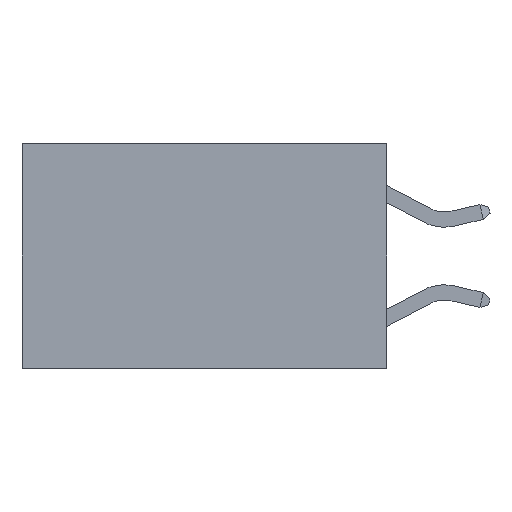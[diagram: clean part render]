
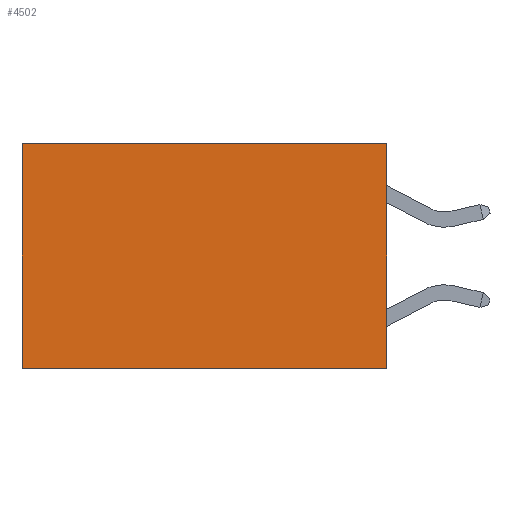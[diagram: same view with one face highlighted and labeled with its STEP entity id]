
A CAD part, left-side view. The second image highlights one B-rep face of the part: STEP entity #4502.
In plain terms, the highlighted planar face has unit normal (-1, 0, 0).
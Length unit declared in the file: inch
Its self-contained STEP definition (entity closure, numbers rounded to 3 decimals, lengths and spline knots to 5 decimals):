
#408 = CARTESIAN_POINT ( 'NONE',  ( 0.2625, 0., 0. ) ) ;
#462 = EDGE_CURVE ( 'NONE', #5724, #863, #1816, .T. ) ;
#844 = CARTESIAN_POINT ( 'NONE',  ( 0.2625, 0., 0. ) ) ;
#863 = VERTEX_POINT ( 'NONE', #2873 ) ;
#1701 = EDGE_CURVE ( 'NONE', #863, #8174, #9578, .T. ) ;
#1816 = LINE ( 'NONE', #408, #9335 ) ;
#1940 = EDGE_LOOP ( 'NONE', ( #2419, #4630, #6530, #8321 ) ) ;
#2263 = DIRECTION ( 'NONE',  ( 0., 0., -1. ) ) ;
#2293 = VECTOR ( 'NONE', #6067, 39.37008 ) ;
#2419 = ORIENTED_EDGE ( 'NONE', *, *, #1701, .T. ) ;
#2873 = CARTESIAN_POINT ( 'NONE',  ( 0.2625, 0.6, 0. ) ) ;
#2953 = VECTOR ( 'NONE', #8441, 39.37008 ) ;
#3237 = LINE ( 'NONE', #4280, #2953 ) ;
#3271 = CARTESIAN_POINT ( 'NONE',  ( 0.2625, 0.6, 0. ) ) ;
#3725 = AXIS2_PLACEMENT_3D ( 'NONE', #9071, #9097, #5076 ) ;
#3895 = CARTESIAN_POINT ( 'NONE',  ( 0.2625, 0., 0. ) ) ;
#3942 = VERTEX_POINT ( 'NONE', #7996 ) ;
#4280 = CARTESIAN_POINT ( 'NONE',  ( 0.2625, 0., -0.37 ) ) ;
#4502 = ADVANCED_FACE ( 'NONE', ( #7821 ), #8464, .F. ) ;
#4533 = LINE ( 'NONE', #3895, #2293 ) ;
#4577 = DIRECTION ( 'NONE',  ( 0., 1., 0. ) ) ;
#4630 = ORIENTED_EDGE ( 'NONE', *, *, #6000, .F. ) ;
#5076 = DIRECTION ( 'NONE',  ( 0., 0., -1. ) ) ;
#5169 = CARTESIAN_POINT ( 'NONE',  ( 0.2625, 0.6, -0.37 ) ) ;
#5724 = VERTEX_POINT ( 'NONE', #844 ) ;
#6000 = EDGE_CURVE ( 'NONE', #3942, #8174, #3237, .T. ) ;
#6064 = VECTOR ( 'NONE', #2263, 39.37008 ) ;
#6067 = DIRECTION ( 'NONE',  ( 0., 0., -1. ) ) ;
#6530 = ORIENTED_EDGE ( 'NONE', *, *, #7644, .F. ) ;
#7644 = EDGE_CURVE ( 'NONE', #5724, #3942, #4533, .T. ) ;
#7821 = FACE_OUTER_BOUND ( 'NONE', #1940, .T. ) ;
#7996 = CARTESIAN_POINT ( 'NONE',  ( 0.2625, 0., -0.37 ) ) ;
#8174 = VERTEX_POINT ( 'NONE', #5169 ) ;
#8321 = ORIENTED_EDGE ( 'NONE', *, *, #462, .T. ) ;
#8441 = DIRECTION ( 'NONE',  ( 0., 1., 0. ) ) ;
#8464 = PLANE ( 'NONE',  #3725 ) ;
#9071 = CARTESIAN_POINT ( 'NONE',  ( 0.2625, 0., 0. ) ) ;
#9097 = DIRECTION ( 'NONE',  ( 1., 0., 0. ) ) ;
#9335 = VECTOR ( 'NONE', #4577, 39.37008 ) ;
#9578 = LINE ( 'NONE', #3271, #6064 ) ;
